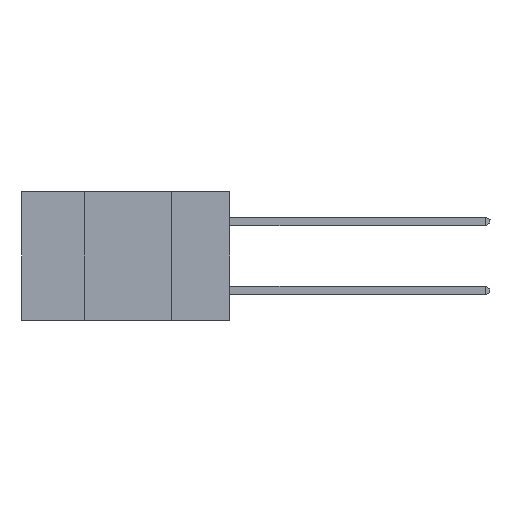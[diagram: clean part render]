
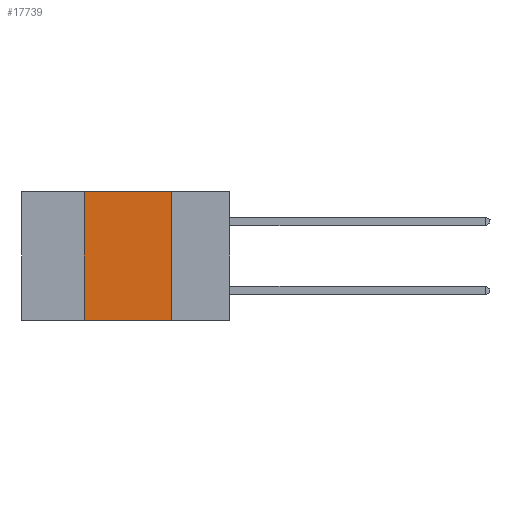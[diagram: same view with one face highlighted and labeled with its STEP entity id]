
A CAD part, left-side view. The second image highlights one B-rep face of the part: STEP entity #17739.
In plain terms, the highlighted planar face has unit normal (-1, 0, 0).
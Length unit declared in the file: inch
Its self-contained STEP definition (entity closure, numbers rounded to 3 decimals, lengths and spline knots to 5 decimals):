
#29 = VERTEX_POINT ( 'NONE', #15010 ) ;
#427 = VERTEX_POINT ( 'NONE', #5803 ) ;
#1039 = LINE ( 'NONE', #3060, #1505 ) ;
#1202 = DIRECTION ( 'NONE',  ( 0., -1., 0. ) ) ;
#1505 = VECTOR ( 'NONE', #6976, 39.37008 ) ;
#1517 = FACE_OUTER_BOUND ( 'NONE', #18253, .T. ) ;
#3060 = CARTESIAN_POINT ( 'NONE',  ( 0., 0.17, -0.37 ) ) ;
#3527 = VECTOR ( 'NONE', #15447, 39.37008 ) ;
#4232 = LINE ( 'NONE', #11932, #14397 ) ;
#5803 = CARTESIAN_POINT ( 'NONE',  ( 0., 0.42, 0. ) ) ;
#6976 = DIRECTION ( 'NONE',  ( 0., 0., -1. ) ) ;
#7541 = CARTESIAN_POINT ( 'NONE',  ( 0., 0.42, -0.37 ) ) ;
#8159 = CARTESIAN_POINT ( 'NONE',  ( 0., 0.6, -0.37 ) ) ;
#8689 = PLANE ( 'NONE',  #16160 ) ;
#9419 = VERTEX_POINT ( 'NONE', #7541 ) ;
#9611 = LINE ( 'NONE', #24677, #3527 ) ;
#11020 = ORIENTED_EDGE ( 'NONE', *, *, #14128, .F. ) ;
#11625 = CARTESIAN_POINT ( 'NONE',  ( 0., 0.17, 0. ) ) ;
#11932 = CARTESIAN_POINT ( 'NONE',  ( 0., 0.6, 0. ) ) ;
#12477 = EDGE_CURVE ( 'NONE', #9419, #29, #13981, .T. ) ;
#13446 = EDGE_CURVE ( 'NONE', #427, #21813, #4232, .T. ) ;
#13981 = LINE ( 'NONE', #8159, #24234 ) ;
#14016 = EDGE_CURVE ( 'NONE', #21813, #29, #1039, .T. ) ;
#14128 = EDGE_CURVE ( 'NONE', #9419, #427, #9611, .T. ) ;
#14397 = VECTOR ( 'NONE', #17896, 39.37008 ) ;
#14780 = CARTESIAN_POINT ( 'NONE',  ( 0., 0.6, 0. ) ) ;
#15010 = CARTESIAN_POINT ( 'NONE',  ( 0., 0.17, -0.37 ) ) ;
#15447 = DIRECTION ( 'NONE',  ( 0., 0., 1. ) ) ;
#15561 = ORIENTED_EDGE ( 'NONE', *, *, #12477, .T. ) ;
#16160 = AXIS2_PLACEMENT_3D ( 'NONE', #14780, #18447, #24522 ) ;
#17739 = ADVANCED_FACE ( 'NONE', ( #1517 ), #8689, .F. ) ;
#17896 = DIRECTION ( 'NONE',  ( 0., -1., 0. ) ) ;
#18253 = EDGE_LOOP ( 'NONE', ( #24061, #18640, #11020, #15561 ) ) ;
#18447 = DIRECTION ( 'NONE',  ( 1., 0., 0. ) ) ;
#18640 = ORIENTED_EDGE ( 'NONE', *, *, #13446, .F. ) ;
#21813 = VERTEX_POINT ( 'NONE', #11625 ) ;
#24061 = ORIENTED_EDGE ( 'NONE', *, *, #14016, .F. ) ;
#24234 = VECTOR ( 'NONE', #1202, 39.37008 ) ;
#24522 = DIRECTION ( 'NONE',  ( 0., 0., -1. ) ) ;
#24677 = CARTESIAN_POINT ( 'NONE',  ( 0., 0.42, -0.37 ) ) ;
